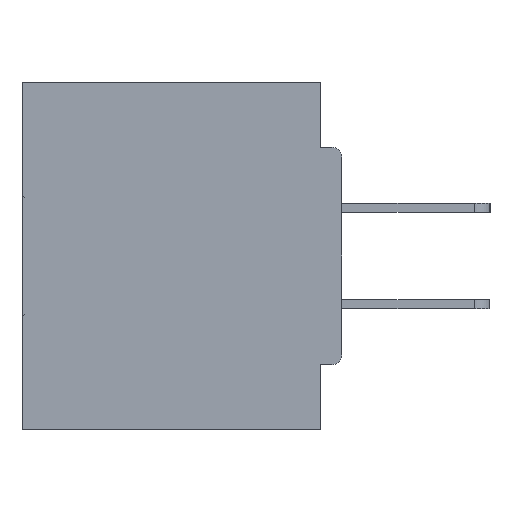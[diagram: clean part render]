
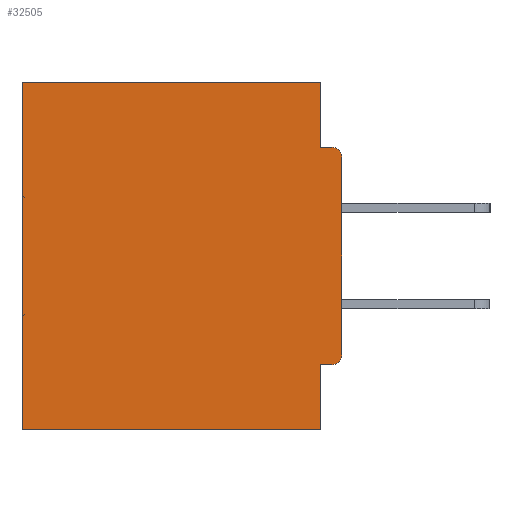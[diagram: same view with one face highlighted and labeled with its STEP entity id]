
A CAD part, left-side view. The second image highlights one B-rep face of the part: STEP entity #32505.
In plain terms, the highlighted planar face has unit normal (-1, 0, 0).
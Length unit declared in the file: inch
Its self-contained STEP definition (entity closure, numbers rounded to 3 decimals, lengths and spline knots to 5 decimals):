
#196 = CARTESIAN_POINT ( 'NONE',  ( 0.298, 0., -0.3915 ) ) ;
#800 = CARTESIAN_POINT ( 'NONE',  ( 0.298, 0.031, 0. ) ) ;
#1419 = ORIENTED_EDGE ( 'NONE', *, *, #18233, .T. ) ;
#2246 = DIRECTION ( 'NONE',  ( 0., 1., 0. ) ) ;
#2341 = ORIENTED_EDGE ( 'NONE', *, *, #6716, .F. ) ;
#2787 = CARTESIAN_POINT ( 'NONE',  ( 0.298, 0., -0.5 ) ) ;
#3011 = ORIENTED_EDGE ( 'NONE', *, *, #28021, .F. ) ;
#3087 = DIRECTION ( 'NONE',  ( 0., 0., -1. ) ) ;
#3823 = VECTOR ( 'NONE', #29653, 39.37008 ) ;
#4434 = CARTESIAN_POINT ( 'NONE',  ( 0.298, 0.031, -0.5 ) ) ;
#6010 = CARTESIAN_POINT ( 'NONE',  ( 0.298, 0.031, -0.0935 ) ) ;
#6256 = ORIENTED_EDGE ( 'NONE', *, *, #18965, .F. ) ;
#6412 = AXIS2_PLACEMENT_3D ( 'NONE', #15923, #39189, #19294 ) ;
#6630 = VERTEX_POINT ( 'NONE', #11024 ) ;
#6669 = CARTESIAN_POINT ( 'NONE',  ( 0.298, 0., 0. ) ) ;
#6710 = CARTESIAN_POINT ( 'NONE',  ( 0.298, 0.015, -0.0935 ) ) ;
#6716 = EDGE_CURVE ( 'NONE', #6630, #9936, #15869, .T. ) ;
#6824 = DIRECTION ( 'NONE',  ( 0., 0., -1. ) ) ;
#8787 = ORIENTED_EDGE ( 'NONE', *, *, #37861, .F. ) ;
#8859 = VERTEX_POINT ( 'NONE', #6010 ) ;
#9110 = EDGE_CURVE ( 'NONE', #6630, #34172, #17944, .T. ) ;
#9936 = VERTEX_POINT ( 'NONE', #12209 ) ;
#10000 = FACE_OUTER_BOUND ( 'NONE', #22154, .T. ) ;
#10328 = EDGE_CURVE ( 'NONE', #9936, #29234, #36566, .T. ) ;
#11024 = CARTESIAN_POINT ( 'NONE',  ( 0.298, 0.015, -0.4065 ) ) ;
#11286 = CARTESIAN_POINT ( 'NONE',  ( 0.298, 0.031, -0.5 ) ) ;
#11415 = VERTEX_POINT ( 'NONE', #16160 ) ;
#11568 = VERTEX_POINT ( 'NONE', #800 ) ;
#11681 = LINE ( 'NONE', #6669, #35638 ) ;
#12209 = CARTESIAN_POINT ( 'NONE',  ( 0.298, 0.031, -0.4065 ) ) ;
#12217 = LINE ( 'NONE', #2787, #13276 ) ;
#12233 = CARTESIAN_POINT ( 'NONE',  ( 0.298, 0.031, -0.5 ) ) ;
#12579 = VECTOR ( 'NONE', #21467, 39.37008 ) ;
#12730 = LINE ( 'NONE', #22973, #3823 ) ;
#13276 = VECTOR ( 'NONE', #30341, 39.37008 ) ;
#13656 = VECTOR ( 'NONE', #34715, 39.37008 ) ;
#13741 = DIRECTION ( 'NONE',  ( -1., 0., 0. ) ) ;
#15671 = ORIENTED_EDGE ( 'NONE', *, *, #33401, .T. ) ;
#15762 = ORIENTED_EDGE ( 'NONE', *, *, #10328, .F. ) ;
#15869 = LINE ( 'NONE', #32257, #38226 ) ;
#15923 = CARTESIAN_POINT ( 'NONE',  ( 0.298, 0.015, -0.1085 ) ) ;
#16160 = CARTESIAN_POINT ( 'NONE',  ( 0.298, 0.46, -0.5 ) ) ;
#17712 = ORIENTED_EDGE ( 'NONE', *, *, #9110, .T. ) ;
#17944 = CIRCLE ( 'NONE', #28195, 0.015 ) ;
#18233 = EDGE_CURVE ( 'NONE', #30304, #21614, #28424, .T. ) ;
#18965 = EDGE_CURVE ( 'NONE', #30304, #34172, #11681, .T. ) ;
#19294 = DIRECTION ( 'NONE',  ( 0., 0., -1. ) ) ;
#20835 = LINE ( 'NONE', #37867, #27600 ) ;
#21467 = DIRECTION ( 'NONE',  ( 0., 0., -1. ) ) ;
#21591 = LINE ( 'NONE', #12233, #24621 ) ;
#21614 = VERTEX_POINT ( 'NONE', #6710 ) ;
#22154 = EDGE_LOOP ( 'NONE', ( #1419, #3011, #39585, #36360, #15671, #8787, #15762, #2341, #17712, #6256 ) ) ;
#22973 = CARTESIAN_POINT ( 'NONE',  ( 0.298, 0., 0. ) ) ;
#23097 = DIRECTION ( 'NONE',  ( 1., 0., 0. ) ) ;
#24621 = VECTOR ( 'NONE', #28421, 39.37008 ) ;
#26402 = CARTESIAN_POINT ( 'NONE',  ( 0.298, 0., -0.1085 ) ) ;
#26641 = CARTESIAN_POINT ( 'NONE',  ( 0.298, 0.46, 0. ) ) ;
#27600 = VECTOR ( 'NONE', #28015, 39.37008 ) ;
#28015 = DIRECTION ( 'NONE',  ( 0., -1., 0. ) ) ;
#28021 = EDGE_CURVE ( 'NONE', #8859, #21614, #20835, .T. ) ;
#28195 = AXIS2_PLACEMENT_3D ( 'NONE', #37131, #13741, #36842 ) ;
#28421 = DIRECTION ( 'NONE',  ( 0., 0., -1. ) ) ;
#28424 = CIRCLE ( 'NONE', #6412, 0.015 ) ;
#29234 = VERTEX_POINT ( 'NONE', #11286 ) ;
#29353 = PLANE ( 'NONE',  #31586 ) ;
#29653 = DIRECTION ( 'NONE',  ( 0., 1., 0. ) ) ;
#30065 = VERTEX_POINT ( 'NONE', #26641 ) ;
#30304 = VERTEX_POINT ( 'NONE', #26402 ) ;
#30341 = DIRECTION ( 'NONE',  ( 0., 1., 0. ) ) ;
#31586 = AXIS2_PLACEMENT_3D ( 'NONE', #36019, #23097, #3087 ) ;
#32257 = CARTESIAN_POINT ( 'NONE',  ( 0.298, 0., -0.4065 ) ) ;
#32505 = ADVANCED_FACE ( 'NONE', ( #10000 ), #29353, .F. ) ;
#33401 = EDGE_CURVE ( 'NONE', #30065, #11415, #38607, .T. ) ;
#34172 = VERTEX_POINT ( 'NONE', #196 ) ;
#34299 = EDGE_CURVE ( 'NONE', #11568, #8859, #21591, .T. ) ;
#34715 = DIRECTION ( 'NONE',  ( 0., 0., -1. ) ) ;
#35638 = VECTOR ( 'NONE', #6824, 39.37008 ) ;
#36019 = CARTESIAN_POINT ( 'NONE',  ( 0.298, 0., 0. ) ) ;
#36360 = ORIENTED_EDGE ( 'NONE', *, *, #42764, .T. ) ;
#36566 = LINE ( 'NONE', #4434, #13656 ) ;
#36842 = DIRECTION ( 'NONE',  ( 0., 0., -1. ) ) ;
#37131 = CARTESIAN_POINT ( 'NONE',  ( 0.298, 0.015, -0.3915 ) ) ;
#37861 = EDGE_CURVE ( 'NONE', #29234, #11415, #12217, .T. ) ;
#37867 = CARTESIAN_POINT ( 'NONE',  ( 0.298, 0., -0.0935 ) ) ;
#38148 = CARTESIAN_POINT ( 'NONE',  ( 0.298, 0.46, 0. ) ) ;
#38226 = VECTOR ( 'NONE', #2246, 39.37008 ) ;
#38607 = LINE ( 'NONE', #38148, #12579 ) ;
#39189 = DIRECTION ( 'NONE',  ( -1., 0., 0. ) ) ;
#39585 = ORIENTED_EDGE ( 'NONE', *, *, #34299, .F. ) ;
#42764 = EDGE_CURVE ( 'NONE', #11568, #30065, #12730, .T. ) ;
